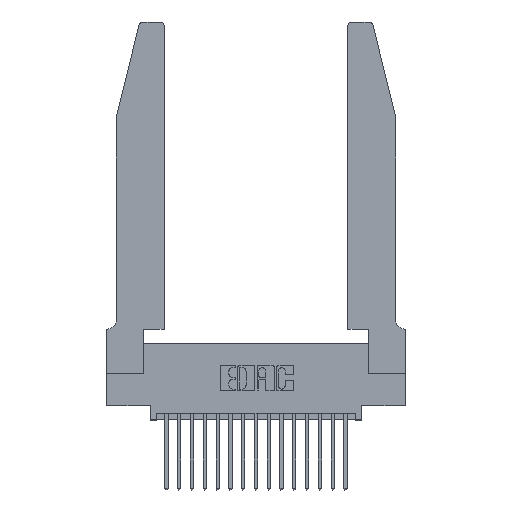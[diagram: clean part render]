
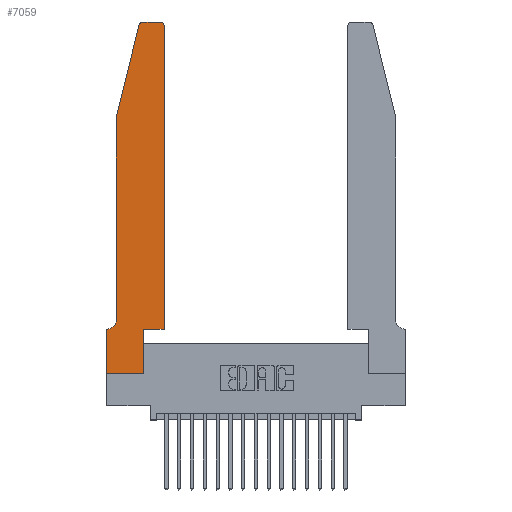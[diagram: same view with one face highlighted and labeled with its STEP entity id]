
A CAD part, top view. The second image highlights one B-rep face of the part: STEP entity #7059.
In plain terms, the highlighted planar face has unit normal (0, 0, 1).
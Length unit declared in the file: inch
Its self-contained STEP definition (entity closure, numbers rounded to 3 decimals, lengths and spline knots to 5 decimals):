
#192 = DIRECTION ( 'NONE',  ( 0., 0., -1. ) ) ;
#372 = VECTOR ( 'NONE', #6312, 39.37008 ) ;
#386 = ORIENTED_EDGE ( 'NONE', *, *, #3725, .T. ) ;
#403 = ORIENTED_EDGE ( 'NONE', *, *, #5960, .T. ) ;
#1224 = VERTEX_POINT ( 'NONE', #18246 ) ;
#1324 = VERTEX_POINT ( 'NONE', #11116 ) ;
#1552 = VECTOR ( 'NONE', #15446, 39.37008 ) ;
#1569 = AXIS2_PLACEMENT_3D ( 'NONE', #9969, #11556, #2039 ) ;
#1698 = CARTESIAN_POINT ( 'NONE',  ( 0.4505, 0.35, 0.37 ) ) ;
#1775 = CARTESIAN_POINT ( 'NONE',  ( 0.2865, 0., 0.37 ) ) ;
#2039 = DIRECTION ( 'NONE',  ( 1., 0., 0. ) ) ;
#2045 = LINE ( 'NONE', #20043, #1552 ) ;
#2422 = VECTOR ( 'NONE', #2606, 39.37008 ) ;
#2606 = DIRECTION ( 'NONE',  ( -1., 0., 0. ) ) ;
#2664 = VECTOR ( 'NONE', #13020, 39.37008 ) ;
#2762 = DIRECTION ( 'NONE',  ( 1., 0., 0. ) ) ;
#2848 = ORIENTED_EDGE ( 'NONE', *, *, #15079, .T. ) ;
#3409 = DIRECTION ( 'NONE',  ( 0., 0., 1. ) ) ;
#3725 = EDGE_CURVE ( 'NONE', #16445, #14398, #9859, .T. ) ;
#3737 = VECTOR ( 'NONE', #8734, 39.37008 ) ;
#4011 = CARTESIAN_POINT ( 'NONE',  ( 0.2865, 0.35, 0.37 ) ) ;
#4095 = DIRECTION ( 'NONE',  ( 0., 0., 1. ) ) ;
#4175 = DIRECTION ( 'NONE',  ( 0., -1., 0. ) ) ;
#4415 = CARTESIAN_POINT ( 'NONE',  ( 0.0755, 0.42, 0.37 ) ) ;
#4616 = LINE ( 'NONE', #16668, #20226 ) ;
#5134 = VERTEX_POINT ( 'NONE', #19159 ) ;
#5154 = CARTESIAN_POINT ( 'NONE',  ( 0.0755, 2., 0.37 ) ) ;
#5184 = EDGE_CURVE ( 'NONE', #5134, #1224, #17025, .T. ) ;
#5265 = DIRECTION ( 'NONE',  ( -1., 0., 0. ) ) ;
#5723 = VERTEX_POINT ( 'NONE', #14507 ) ;
#5960 = EDGE_CURVE ( 'NONE', #1324, #5134, #16267, .T. ) ;
#6312 = DIRECTION ( 'NONE',  ( 1., 0., 0. ) ) ;
#6327 = EDGE_CURVE ( 'NONE', #1224, #9928, #17684, .T. ) ;
#6934 = VECTOR ( 'NONE', #2762, 39.37008 ) ;
#7059 = ADVANCED_FACE ( 'NONE', ( #17426 ), #19196, .T. ) ;
#7334 = VERTEX_POINT ( 'NONE', #4415 ) ;
#7793 = ORIENTED_EDGE ( 'NONE', *, *, #5184, .T. ) ;
#7931 = CARTESIAN_POINT ( 'NONE',  ( 0.4505, 0.35, 0.37 ) ) ;
#7981 = LINE ( 'NONE', #14820, #3737 ) ;
#8619 = EDGE_CURVE ( 'NONE', #5723, #9762, #14736, .T. ) ;
#8734 = DIRECTION ( 'NONE',  ( 0., 1., 0. ) ) ;
#9546 = ORIENTED_EDGE ( 'NONE', *, *, #18305, .T. ) ;
#9747 = CARTESIAN_POINT ( 'NONE',  ( 0.0055, 0.42, 0.37 ) ) ;
#9762 = VERTEX_POINT ( 'NONE', #1775 ) ;
#9859 = LINE ( 'NONE', #7931, #372 ) ;
#9928 = VERTEX_POINT ( 'NONE', #17837 ) ;
#9969 = CARTESIAN_POINT ( 'NONE',  ( 0., 0.35, 0.37 ) ) ;
#10092 = EDGE_CURVE ( 'NONE', #14309, #19962, #10387, .T. ) ;
#10323 = VECTOR ( 'NONE', #18651, 39.37008 ) ;
#10387 = LINE ( 'NONE', #16715, #2422 ) ;
#10622 = AXIS2_PLACEMENT_3D ( 'NONE', #13505, #4095, #15047 ) ;
#11116 = CARTESIAN_POINT ( 'NONE',  ( 0.4505, 2.72, 0.37 ) ) ;
#11260 = VERTEX_POINT ( 'NONE', #15055 ) ;
#11330 = DIRECTION ( 'NONE',  ( -1., 0., 0. ) ) ;
#11512 = EDGE_CURVE ( 'NONE', #9928, #11260, #18494, .T. ) ;
#11543 = ORIENTED_EDGE ( 'NONE', *, *, #8619, .T. ) ;
#11556 = DIRECTION ( 'NONE',  ( 0., 0., 1. ) ) ;
#12483 = VECTOR ( 'NONE', #5265, 39.37008 ) ;
#12867 = CARTESIAN_POINT ( 'NONE',  ( 0.284, 2.72, 0.37 ) ) ;
#12969 = EDGE_LOOP ( 'NONE', ( #7793, #13895, #19595, #2848, #9546, #17817, #18962, #11543, #15611, #386, #20052, #403 ) ) ;
#13020 = DIRECTION ( 'NONE',  ( 0., -1., 0. ) ) ;
#13071 = CARTESIAN_POINT ( 'NONE',  ( 0.2605, 2.75, 0.37 ) ) ;
#13505 = CARTESIAN_POINT ( 'NONE',  ( 0.4205, 2.72, 0.37 ) ) ;
#13782 = CARTESIAN_POINT ( 'NONE',  ( 0., 0., 0.37 ) ) ;
#13895 = ORIENTED_EDGE ( 'NONE', *, *, #6327, .T. ) ;
#14042 = CARTESIAN_POINT ( 'NONE',  ( 0.0755, 2., 0.37 ) ) ;
#14089 = CIRCLE ( 'NONE', #17615, 0.07 ) ;
#14309 = VERTEX_POINT ( 'NONE', #15670 ) ;
#14392 = DIRECTION ( 'NONE',  ( 1., 0., 0. ) ) ;
#14398 = VERTEX_POINT ( 'NONE', #1698 ) ;
#14507 = CARTESIAN_POINT ( 'NONE',  ( 0., 0., 0.37 ) ) ;
#14673 = EDGE_CURVE ( 'NONE', #14398, #1324, #7981, .T. ) ;
#14736 = LINE ( 'NONE', #13782, #6934 ) ;
#14820 = CARTESIAN_POINT ( 'NONE',  ( 0.4505, 0.35, 0.37 ) ) ;
#15047 = DIRECTION ( 'NONE',  ( 1., 0., 0. ) ) ;
#15055 = CARTESIAN_POINT ( 'NONE',  ( 0.0755, 2., 0.37 ) ) ;
#15079 = EDGE_CURVE ( 'NONE', #11260, #7334, #18773, .T. ) ;
#15446 = DIRECTION ( 'NONE',  ( 0., 1., 0. ) ) ;
#15611 = ORIENTED_EDGE ( 'NONE', *, *, #17398, .T. ) ;
#15670 = CARTESIAN_POINT ( 'NONE',  ( 0.0055, 0.35, 0.37 ) ) ;
#15940 = EDGE_CURVE ( 'NONE', #19962, #5723, #4616, .T. ) ;
#16267 = CIRCLE ( 'NONE', #10622, 0.03 ) ;
#16445 = VERTEX_POINT ( 'NONE', #4011 ) ;
#16668 = CARTESIAN_POINT ( 'NONE',  ( 0., 0., 0.37 ) ) ;
#16715 = CARTESIAN_POINT ( 'NONE',  ( 0.0755, 0.35, 0.37 ) ) ;
#17025 = LINE ( 'NONE', #13071, #12483 ) ;
#17398 = EDGE_CURVE ( 'NONE', #9762, #16445, #2045, .T. ) ;
#17426 = FACE_OUTER_BOUND ( 'NONE', #12969, .T. ) ;
#17615 = AXIS2_PLACEMENT_3D ( 'NONE', #9747, #192, #11330 ) ;
#17684 = CIRCLE ( 'NONE', #18457, 0.03 ) ;
#17817 = ORIENTED_EDGE ( 'NONE', *, *, #10092, .T. ) ;
#17837 = CARTESIAN_POINT ( 'NONE',  ( 0.25487, 2.72718, 0.37 ) ) ;
#18246 = CARTESIAN_POINT ( 'NONE',  ( 0.284, 2.75, 0.37 ) ) ;
#18305 = EDGE_CURVE ( 'NONE', #7334, #14309, #14089, .T. ) ;
#18457 = AXIS2_PLACEMENT_3D ( 'NONE', #12867, #3409, #14392 ) ;
#18494 = LINE ( 'NONE', #14042, #10323 ) ;
#18651 = DIRECTION ( 'NONE',  ( -0.239, -0.971, 0. ) ) ;
#18773 = LINE ( 'NONE', #5154, #2664 ) ;
#18962 = ORIENTED_EDGE ( 'NONE', *, *, #15940, .T. ) ;
#19159 = CARTESIAN_POINT ( 'NONE',  ( 0.4205, 2.75, 0.37 ) ) ;
#19196 = PLANE ( 'NONE',  #1569 ) ;
#19277 = CARTESIAN_POINT ( 'NONE',  ( 0., 0.35, 0.37 ) ) ;
#19595 = ORIENTED_EDGE ( 'NONE', *, *, #11512, .T. ) ;
#19962 = VERTEX_POINT ( 'NONE', #19277 ) ;
#20043 = CARTESIAN_POINT ( 'NONE',  ( 0.2865, 0.35, 0.37 ) ) ;
#20052 = ORIENTED_EDGE ( 'NONE', *, *, #14673, .T. ) ;
#20226 = VECTOR ( 'NONE', #4175, 39.37008 ) ;
